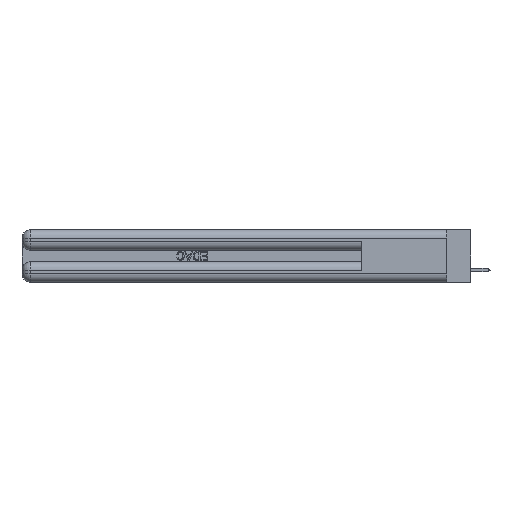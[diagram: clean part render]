
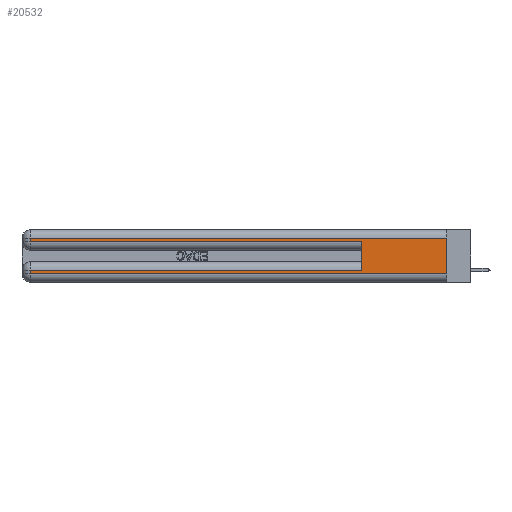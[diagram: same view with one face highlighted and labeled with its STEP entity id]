
A CAD part, left-side view. The second image highlights one B-rep face of the part: STEP entity #20532.
In plain terms, the highlighted planar face has unit normal (-1, 0, 0).
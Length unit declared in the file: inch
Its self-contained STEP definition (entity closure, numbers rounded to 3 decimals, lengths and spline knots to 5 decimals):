
#162 = CARTESIAN_POINT ( 'NONE',  ( 0., 2.94, 0.06 ) ) ;
#922 = DIRECTION ( 'NONE',  ( 0., 0., -1. ) ) ;
#1011 = CARTESIAN_POINT ( 'NONE',  ( 0., 0., 0.37 ) ) ;
#1512 = ORIENTED_EDGE ( 'NONE', *, *, #34382, .F. ) ;
#2893 = FACE_OUTER_BOUND ( 'NONE', #9787, .T. ) ;
#4116 = LINE ( 'NONE', #37652, #11580 ) ;
#4430 = DIRECTION ( 'NONE',  ( 0., 0., -1. ) ) ;
#6291 = CARTESIAN_POINT ( 'NONE',  ( 0., 2.94, 0.31 ) ) ;
#7187 = VERTEX_POINT ( 'NONE', #12125 ) ;
#7329 = LINE ( 'NONE', #36026, #11545 ) ;
#8370 = VERTEX_POINT ( 'NONE', #162 ) ;
#9494 = DIRECTION ( 'NONE',  ( 0., 0., 1. ) ) ;
#9694 = LINE ( 'NONE', #21324, #21917 ) ;
#9787 = EDGE_LOOP ( 'NONE', ( #22814, #27807, #22910, #23924, #1512, #37908, #32523, #36898 ) ) ;
#10865 = CARTESIAN_POINT ( 'NONE',  ( 0., 0.6, 0.085 ) ) ;
#10877 = CARTESIAN_POINT ( 'NONE',  ( 0., 2.94, 0.085 ) ) ;
#11375 = VERTEX_POINT ( 'NONE', #25637 ) ;
#11472 = EDGE_CURVE ( 'NONE', #7187, #26051, #7329, .T. ) ;
#11545 = VECTOR ( 'NONE', #922, 39.37008 ) ;
#11580 = VECTOR ( 'NONE', #4430, 39.37008 ) ;
#12125 = CARTESIAN_POINT ( 'NONE',  ( 0., 0., 0.31 ) ) ;
#12355 = DIRECTION ( 'NONE',  ( 0., 1., 0. ) ) ;
#12686 = EDGE_CURVE ( 'NONE', #11375, #16455, #31578, .T. ) ;
#13212 = AXIS2_PLACEMENT_3D ( 'NONE', #1011, #16104, #28020 ) ;
#13333 = DIRECTION ( 'NONE',  ( 0., 1., 0. ) ) ;
#13761 = EDGE_CURVE ( 'NONE', #8370, #26051, #29845, .T. ) ;
#14457 = CARTESIAN_POINT ( 'NONE',  ( 0., 0., 0.285 ) ) ;
#14776 = VERTEX_POINT ( 'NONE', #10877 ) ;
#16104 = DIRECTION ( 'NONE',  ( 1., 0., 0. ) ) ;
#16447 = DIRECTION ( 'NONE',  ( 0., -1., 0. ) ) ;
#16455 = VERTEX_POINT ( 'NONE', #27625 ) ;
#16977 = LINE ( 'NONE', #23424, #30998 ) ;
#18643 = VECTOR ( 'NONE', #16447, 39.37008 ) ;
#19283 = CARTESIAN_POINT ( 'NONE',  ( 0., 0., 0.085 ) ) ;
#20257 = VECTOR ( 'NONE', #13333, 39.37008 ) ;
#20532 = ADVANCED_FACE ( 'NONE', ( #2893 ), #27896, .F. ) ;
#20714 = EDGE_CURVE ( 'NONE', #25307, #11375, #16977, .T. ) ;
#21184 = LINE ( 'NONE', #19283, #20257 ) ;
#21324 = CARTESIAN_POINT ( 'NONE',  ( 0., 0., 0.31 ) ) ;
#21917 = VECTOR ( 'NONE', #12355, 39.37008 ) ;
#21972 = VECTOR ( 'NONE', #9494, 39.37008 ) ;
#22109 = CARTESIAN_POINT ( 'NONE',  ( 0., 0., 0.06 ) ) ;
#22814 = ORIENTED_EDGE ( 'NONE', *, *, #11472, .F. ) ;
#22910 = ORIENTED_EDGE ( 'NONE', *, *, #20714, .T. ) ;
#23424 = CARTESIAN_POINT ( 'NONE',  ( 0., 2.94, 0.37 ) ) ;
#23924 = ORIENTED_EDGE ( 'NONE', *, *, #12686, .T. ) ;
#24607 = EDGE_CURVE ( 'NONE', #7187, #25307, #9694, .T. ) ;
#25307 = VERTEX_POINT ( 'NONE', #6291 ) ;
#25454 = VERTEX_POINT ( 'NONE', #10865 ) ;
#25637 = CARTESIAN_POINT ( 'NONE',  ( 0., 2.94, 0.285 ) ) ;
#26051 = VERTEX_POINT ( 'NONE', #37498 ) ;
#26535 = DIRECTION ( 'NONE',  ( 0., -1., 0. ) ) ;
#27625 = CARTESIAN_POINT ( 'NONE',  ( 0., 0.6, 0.285 ) ) ;
#27807 = ORIENTED_EDGE ( 'NONE', *, *, #24607, .T. ) ;
#27896 = PLANE ( 'NONE',  #13212 ) ;
#28020 = DIRECTION ( 'NONE',  ( 0., 0., -1. ) ) ;
#29845 = LINE ( 'NONE', #22109, #18643 ) ;
#30884 = EDGE_CURVE ( 'NONE', #14776, #8370, #4116, .T. ) ;
#30974 = CARTESIAN_POINT ( 'NONE',  ( 0., 0.6, 0.145 ) ) ;
#30998 = VECTOR ( 'NONE', #38401, 39.37008 ) ;
#31578 = LINE ( 'NONE', #14457, #32067 ) ;
#32067 = VECTOR ( 'NONE', #26535, 39.37008 ) ;
#32523 = ORIENTED_EDGE ( 'NONE', *, *, #30884, .T. ) ;
#32692 = EDGE_CURVE ( 'NONE', #25454, #14776, #21184, .T. ) ;
#34382 = EDGE_CURVE ( 'NONE', #25454, #16455, #37822, .T. ) ;
#36026 = CARTESIAN_POINT ( 'NONE',  ( 0., 0., 0.37 ) ) ;
#36898 = ORIENTED_EDGE ( 'NONE', *, *, #13761, .T. ) ;
#37498 = CARTESIAN_POINT ( 'NONE',  ( 0., 0., 0.06 ) ) ;
#37652 = CARTESIAN_POINT ( 'NONE',  ( 0., 2.94, 0.37 ) ) ;
#37822 = LINE ( 'NONE', #30974, #21972 ) ;
#37908 = ORIENTED_EDGE ( 'NONE', *, *, #32692, .T. ) ;
#38401 = DIRECTION ( 'NONE',  ( 0., 0., -1. ) ) ;
